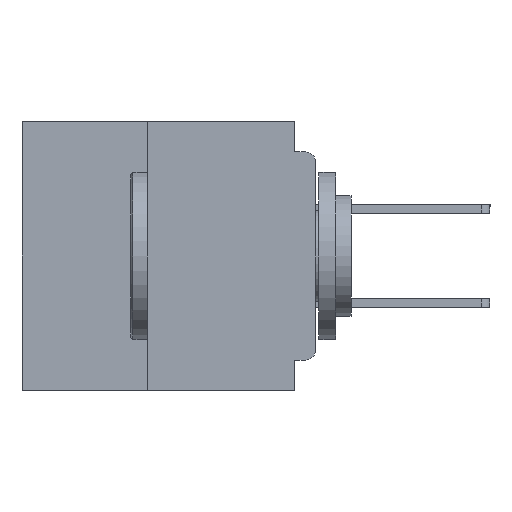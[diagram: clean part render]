
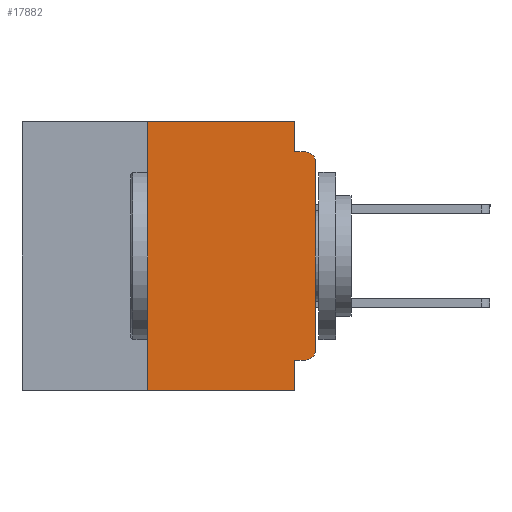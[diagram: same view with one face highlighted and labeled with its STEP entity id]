
A CAD part, left-side view. The second image highlights one B-rep face of the part: STEP entity #17882.
In plain terms, the highlighted planar face has unit normal (-1, 0, 0).
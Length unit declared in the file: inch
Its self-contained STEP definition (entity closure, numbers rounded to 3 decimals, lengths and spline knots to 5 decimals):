
#236 = DIRECTION ( 'NONE',  ( -1., 0., 0. ) ) ;
#401 = VERTEX_POINT ( 'NONE', #24054 ) ;
#1339 = VECTOR ( 'NONE', #17176, 39.37008 ) ;
#1955 = CARTESIAN_POINT ( 'NONE',  ( 0., 0., 0. ) ) ;
#2213 = EDGE_CURVE ( 'NONE', #46770, #57235, #9549, .T. ) ;
#2714 = ORIENTED_EDGE ( 'NONE', *, *, #47117, .F. ) ;
#3102 = LINE ( 'NONE', #21268, #13636 ) ;
#3658 = CARTESIAN_POINT ( 'NONE',  ( 0., 0.031, 0. ) ) ;
#4030 = CARTESIAN_POINT ( 'NONE',  ( 0., 0.031, -0.4 ) ) ;
#4182 = LINE ( 'NONE', #3658, #1339 ) ;
#4428 = DIRECTION ( 'NONE',  ( 0., -1., 0. ) ) ;
#5709 = CARTESIAN_POINT ( 'NONE',  ( 0., 0.437, -0.4 ) ) ;
#6607 = DIRECTION ( 'NONE',  ( 1., 0., 0. ) ) ;
#6836 = CARTESIAN_POINT ( 'NONE',  ( 0., 0., -0.06 ) ) ;
#7358 = ORIENTED_EDGE ( 'NONE', *, *, #20850, .T. ) ;
#7928 = EDGE_CURVE ( 'NONE', #401, #34883, #46757, .T. ) ;
#8959 = CARTESIAN_POINT ( 'NONE',  ( 0., 0., -0.045 ) ) ;
#9549 = CIRCLE ( 'NONE', #27740, 0.015 ) ;
#9566 = VECTOR ( 'NONE', #4428, 39.37008 ) ;
#13209 = DIRECTION ( 'NONE',  ( 0., 0., 1. ) ) ;
#13386 = CARTESIAN_POINT ( 'NONE',  ( 0., 0.25, 0. ) ) ;
#13636 = VECTOR ( 'NONE', #34512, 39.37008 ) ;
#13870 = VECTOR ( 'NONE', #33017, 39.37008 ) ;
#15361 = CARTESIAN_POINT ( 'NONE',  ( 0., 0.015, -0.045 ) ) ;
#15445 = PLANE ( 'NONE',  #25266 ) ;
#16060 = LINE ( 'NONE', #39151, #49761 ) ;
#16600 = VERTEX_POINT ( 'NONE', #54552 ) ;
#17176 = DIRECTION ( 'NONE',  ( 0., 0., -1. ) ) ;
#17882 = ADVANCED_FACE ( 'NONE', ( #48105 ), #15445, .F. ) ;
#19086 = CARTESIAN_POINT ( 'NONE',  ( 0., 0.031, -0.4 ) ) ;
#19283 = LINE ( 'NONE', #4030, #52897 ) ;
#19506 = EDGE_LOOP ( 'NONE', ( #30703, #41236, #2714, #37592, #54825, #28138, #7358, #37043, #33867, #55750 ) ) ;
#19997 = EDGE_CURVE ( 'NONE', #29476, #30626, #29763, .T. ) ;
#20157 = VERTEX_POINT ( 'NONE', #19086 ) ;
#20850 = EDGE_CURVE ( 'NONE', #401, #20157, #44145, .T. ) ;
#21268 = CARTESIAN_POINT ( 'NONE',  ( 0., 0., -0.355 ) ) ;
#21371 = LINE ( 'NONE', #8959, #9566 ) ;
#22386 = AXIS2_PLACEMENT_3D ( 'NONE', #26989, #236, #31346 ) ;
#23596 = DIRECTION ( 'NONE',  ( 0., -1., 0. ) ) ;
#24054 = CARTESIAN_POINT ( 'NONE',  ( 0., 0.25, -0.4 ) ) ;
#25266 = AXIS2_PLACEMENT_3D ( 'NONE', #55000, #6607, #37611 ) ;
#25618 = LINE ( 'NONE', #1955, #13870 ) ;
#26989 = CARTESIAN_POINT ( 'NONE',  ( 0., 0.015, -0.06 ) ) ;
#27740 = AXIS2_PLACEMENT_3D ( 'NONE', #46591, #46546, #46477 ) ;
#27989 = CARTESIAN_POINT ( 'NONE',  ( 0., 0.031, -0.355 ) ) ;
#28097 = CARTESIAN_POINT ( 'NONE',  ( 0., 0., -0.34 ) ) ;
#28138 = ORIENTED_EDGE ( 'NONE', *, *, #7928, .F. ) ;
#29476 = VERTEX_POINT ( 'NONE', #6836 ) ;
#29763 = CIRCLE ( 'NONE', #22386, 0.015 ) ;
#30626 = VERTEX_POINT ( 'NONE', #15361 ) ;
#30703 = ORIENTED_EDGE ( 'NONE', *, *, #35180, .T. ) ;
#31346 = DIRECTION ( 'NONE',  ( 0., 0., -1. ) ) ;
#31504 = EDGE_CURVE ( 'NONE', #46770, #31851, #3102, .T. ) ;
#31851 = VERTEX_POINT ( 'NONE', #27989 ) ;
#33017 = DIRECTION ( 'NONE',  ( 0., 0., 1. ) ) ;
#33334 = CARTESIAN_POINT ( 'NONE',  ( 0., 0.015, -0.355 ) ) ;
#33867 = ORIENTED_EDGE ( 'NONE', *, *, #31504, .F. ) ;
#34094 = EDGE_CURVE ( 'NONE', #16600, #34496, #4182, .T. ) ;
#34496 = VERTEX_POINT ( 'NONE', #50371 ) ;
#34512 = DIRECTION ( 'NONE',  ( 0., 1., 0. ) ) ;
#34674 = DIRECTION ( 'NONE',  ( 0., -1., 0. ) ) ;
#34883 = VERTEX_POINT ( 'NONE', #13386 ) ;
#35180 = EDGE_CURVE ( 'NONE', #57235, #29476, #25618, .T. ) ;
#37043 = ORIENTED_EDGE ( 'NONE', *, *, #40148, .F. ) ;
#37592 = ORIENTED_EDGE ( 'NONE', *, *, #34094, .F. ) ;
#37611 = DIRECTION ( 'NONE',  ( 0., 0., -1. ) ) ;
#39151 = CARTESIAN_POINT ( 'NONE',  ( 0., 0.437, 0. ) ) ;
#40148 = EDGE_CURVE ( 'NONE', #31851, #20157, #19283, .T. ) ;
#41236 = ORIENTED_EDGE ( 'NONE', *, *, #19997, .T. ) ;
#44047 = CARTESIAN_POINT ( 'NONE',  ( 0., 0.25, -0.4 ) ) ;
#44145 = LINE ( 'NONE', #5709, #45529 ) ;
#45529 = VECTOR ( 'NONE', #23596, 39.37008 ) ;
#46477 = DIRECTION ( 'NONE',  ( 0., 0., -1. ) ) ;
#46546 = DIRECTION ( 'NONE',  ( -1., 0., 0. ) ) ;
#46591 = CARTESIAN_POINT ( 'NONE',  ( 0., 0.015, -0.34 ) ) ;
#46757 = LINE ( 'NONE', #44047, #56968 ) ;
#46770 = VERTEX_POINT ( 'NONE', #33334 ) ;
#47117 = EDGE_CURVE ( 'NONE', #34496, #30626, #21371, .T. ) ;
#48105 = FACE_OUTER_BOUND ( 'NONE', #19506, .T. ) ;
#49761 = VECTOR ( 'NONE', #34674, 39.37008 ) ;
#50371 = CARTESIAN_POINT ( 'NONE',  ( 0., 0.031, -0.045 ) ) ;
#52897 = VECTOR ( 'NONE', #56858, 39.37008 ) ;
#54552 = CARTESIAN_POINT ( 'NONE',  ( 0., 0.031, 0. ) ) ;
#54825 = ORIENTED_EDGE ( 'NONE', *, *, #56246, .F. ) ;
#55000 = CARTESIAN_POINT ( 'NONE',  ( 0., 0.437, 0. ) ) ;
#55750 = ORIENTED_EDGE ( 'NONE', *, *, #2213, .T. ) ;
#56246 = EDGE_CURVE ( 'NONE', #34883, #16600, #16060, .T. ) ;
#56858 = DIRECTION ( 'NONE',  ( 0., 0., -1. ) ) ;
#56968 = VECTOR ( 'NONE', #13209, 39.37008 ) ;
#57235 = VERTEX_POINT ( 'NONE', #28097 ) ;
